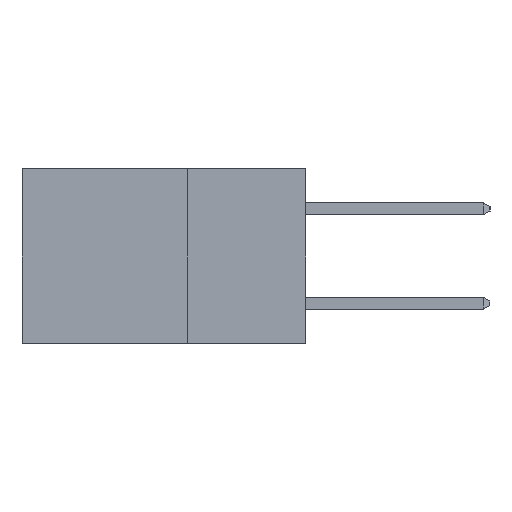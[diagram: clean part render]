
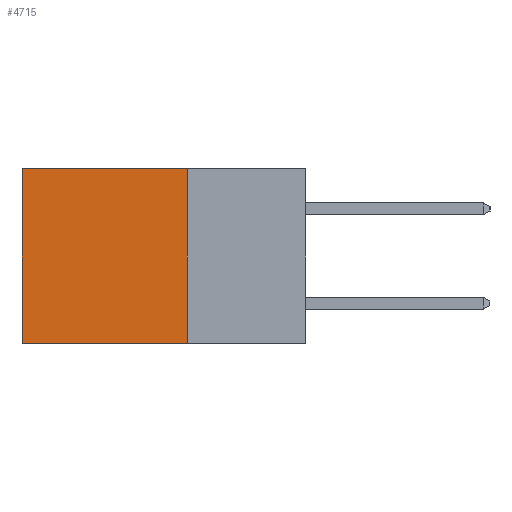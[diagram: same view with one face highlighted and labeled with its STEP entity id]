
A CAD part, left-side view. The second image highlights one B-rep face of the part: STEP entity #4715.
In plain terms, the highlighted planar face has unit normal (-1, 0, 0).
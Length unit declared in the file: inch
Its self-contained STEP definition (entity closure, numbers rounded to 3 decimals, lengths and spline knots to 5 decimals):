
#299 = CARTESIAN_POINT ( 'NONE',  ( 0.2615, 0.25, -0.37 ) ) ;
#1514 = EDGE_CURVE ( 'NONE', #15045, #20643, #8377, .T. ) ;
#1937 = VERTEX_POINT ( 'NONE', #9727 ) ;
#2539 = CARTESIAN_POINT ( 'NONE',  ( 0.2615, 0.6, -0.37 ) ) ;
#2699 = FACE_OUTER_BOUND ( 'NONE', #11452, .T. ) ;
#2755 = VECTOR ( 'NONE', #17131, 39.37008 ) ;
#2851 = CARTESIAN_POINT ( 'NONE',  ( 0.2615, 0.25, 0. ) ) ;
#3755 = LINE ( 'NONE', #2539, #8417 ) ;
#3920 = ORIENTED_EDGE ( 'NONE', *, *, #16859, .F. ) ;
#4682 = DIRECTION ( 'NONE',  ( 0., 1., 0. ) ) ;
#4715 = ADVANCED_FACE ( 'NONE', ( #2699 ), #12903, .F. ) ;
#6045 = DIRECTION ( 'NONE',  ( 1., 0., 0. ) ) ;
#6698 = AXIS2_PLACEMENT_3D ( 'NONE', #14615, #6045, #18014 ) ;
#6798 = EDGE_CURVE ( 'NONE', #1937, #14951, #3755, .T. ) ;
#7591 = ORIENTED_EDGE ( 'NONE', *, *, #6798, .T. ) ;
#8377 = LINE ( 'NONE', #299, #16920 ) ;
#8417 = VECTOR ( 'NONE', #13017, 39.37008 ) ;
#8635 = LINE ( 'NONE', #2851, #22269 ) ;
#8873 = CARTESIAN_POINT ( 'NONE',  ( 0.2615, 0.6, -0.37 ) ) ;
#9258 = EDGE_CURVE ( 'NONE', #15045, #1937, #8635, .T. ) ;
#9727 = CARTESIAN_POINT ( 'NONE',  ( 0.2615, 0.6, 0. ) ) ;
#10692 = ORIENTED_EDGE ( 'NONE', *, *, #9258, .T. ) ;
#11452 = EDGE_LOOP ( 'NONE', ( #7591, #3920, #18423, #10692 ) ) ;
#12903 = PLANE ( 'NONE',  #6698 ) ;
#13017 = DIRECTION ( 'NONE',  ( 0., 0., -1. ) ) ;
#14615 = CARTESIAN_POINT ( 'NONE',  ( 0.2615, 0.25, -0.37 ) ) ;
#14951 = VERTEX_POINT ( 'NONE', #8873 ) ;
#15045 = VERTEX_POINT ( 'NONE', #20955 ) ;
#15444 = CARTESIAN_POINT ( 'NONE',  ( 0.2615, 0.25, -0.37 ) ) ;
#16859 = EDGE_CURVE ( 'NONE', #20643, #14951, #20589, .T. ) ;
#16920 = VECTOR ( 'NONE', #21514, 39.37008 ) ;
#17131 = DIRECTION ( 'NONE',  ( 0., 1., 0. ) ) ;
#18014 = DIRECTION ( 'NONE',  ( 0., 0., -1. ) ) ;
#18092 = CARTESIAN_POINT ( 'NONE',  ( 0.2615, 0.25, -0.37 ) ) ;
#18423 = ORIENTED_EDGE ( 'NONE', *, *, #1514, .F. ) ;
#20589 = LINE ( 'NONE', #15444, #2755 ) ;
#20643 = VERTEX_POINT ( 'NONE', #18092 ) ;
#20955 = CARTESIAN_POINT ( 'NONE',  ( 0.2615, 0.25, 0. ) ) ;
#21514 = DIRECTION ( 'NONE',  ( 0., 0., -1. ) ) ;
#22269 = VECTOR ( 'NONE', #4682, 39.37008 ) ;
